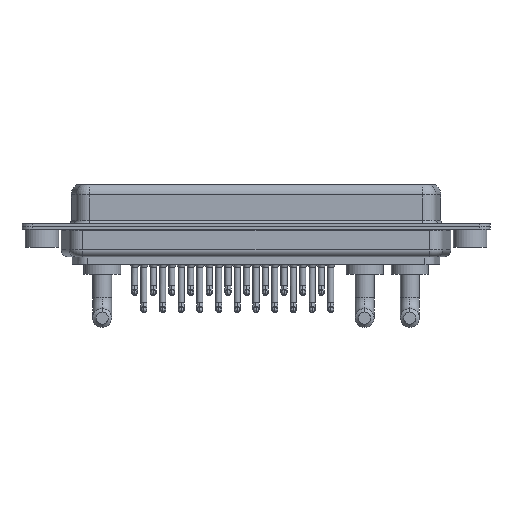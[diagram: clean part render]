
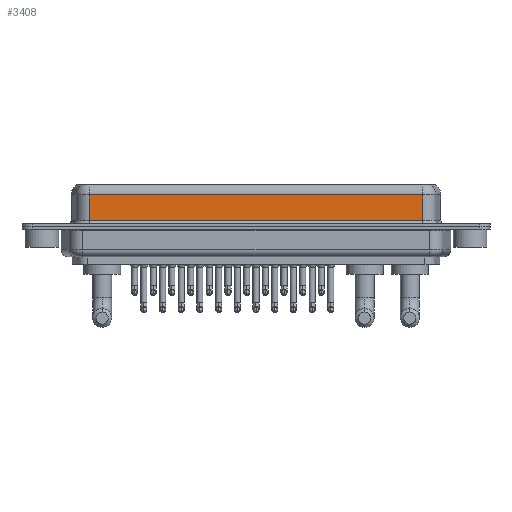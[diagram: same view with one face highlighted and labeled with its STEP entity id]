
A CAD part, front view. The second image highlights one B-rep face of the part: STEP entity #3408.
In plain terms, the highlighted planar face has unit normal (0, -1, 0).
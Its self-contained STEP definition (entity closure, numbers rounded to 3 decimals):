
#1610 = EDGE_CURVE ( 'NONE', #9133, #15918, #8684, .T. ) ;
#2020 = VECTOR ( 'NONE', #16009, 1000. ) ;
#2879 = CARTESIAN_POINT ( 'NONE',  ( 56.462, -3.95, 6.4 ) ) ;
#3000 = DIRECTION ( 'NONE',  ( 0., 0., 1. ) ) ;
#3408 = ADVANCED_FACE ( 'NONE', ( #19494 ), #6609, .F. ) ;
#3452 = CARTESIAN_POINT ( 'NONE',  ( 56.462, -3.95, 4.65 ) ) ;
#4137 = DIRECTION ( 'NONE',  ( 0., 0., -1. ) ) ;
#5149 = LINE ( 'NONE', #3452, #11398 ) ;
#5244 = ORIENTED_EDGE ( 'NONE', *, *, #19730, .F. ) ;
#5341 = EDGE_CURVE ( 'NONE', #6265, #8928, #5149, .T. ) ;
#6265 = VERTEX_POINT ( 'NONE', #6777 ) ;
#6609 = PLANE ( 'NONE',  #21312 ) ;
#6777 = CARTESIAN_POINT ( 'NONE',  ( 56.462, -3.95, 4.65 ) ) ;
#7071 = DIRECTION ( 'NONE',  ( -1., 0., 0. ) ) ;
#7263 = ORIENTED_EDGE ( 'NONE', *, *, #1610, .T. ) ;
#7664 = ORIENTED_EDGE ( 'NONE', *, *, #5341, .T. ) ;
#8684 = LINE ( 'NONE', #23245, #2020 ) ;
#8928 = VERTEX_POINT ( 'NONE', #9220 ) ;
#9133 = VERTEX_POINT ( 'NONE', #9928 ) ;
#9220 = CARTESIAN_POINT ( 'NONE',  ( 7.038, -3.95, 4.65 ) ) ;
#9928 = CARTESIAN_POINT ( 'NONE',  ( 7.038, -3.95, 0.9 ) ) ;
#10221 = DIRECTION ( 'NONE',  ( 0., 1., 0. ) ) ;
#10499 = CARTESIAN_POINT ( 'NONE',  ( 7.038, -3.95, 6.4 ) ) ;
#11398 = VECTOR ( 'NONE', #7071, 1000. ) ;
#14219 = EDGE_LOOP ( 'NONE', ( #5244, #7664, #14256, #7263 ) ) ;
#14256 = ORIENTED_EDGE ( 'NONE', *, *, #16415, .T. ) ;
#14329 = DIRECTION ( 'NONE',  ( 0., 0., -1. ) ) ;
#15918 = VERTEX_POINT ( 'NONE', #22236 ) ;
#16009 = DIRECTION ( 'NONE',  ( 1., 0., 0. ) ) ;
#16025 = LINE ( 'NONE', #10499, #22560 ) ;
#16415 = EDGE_CURVE ( 'NONE', #8928, #9133, #16025, .T. ) ;
#18063 = VECTOR ( 'NONE', #4137, 1000. ) ;
#19494 = FACE_OUTER_BOUND ( 'NONE', #14219, .T. ) ;
#19730 = EDGE_CURVE ( 'NONE', #6265, #15918, #20632, .T. ) ;
#20394 = CARTESIAN_POINT ( 'NONE',  ( 56.462, -3.95, 6.4 ) ) ;
#20632 = LINE ( 'NONE', #20394, #18063 ) ;
#21312 = AXIS2_PLACEMENT_3D ( 'NONE', #2879, #10221, #3000 ) ;
#22236 = CARTESIAN_POINT ( 'NONE',  ( 56.462, -3.95, 0.9 ) ) ;
#22560 = VECTOR ( 'NONE', #14329, 1000. ) ;
#23245 = CARTESIAN_POINT ( 'NONE',  ( 56.462, -3.95, 0.9 ) ) ;
